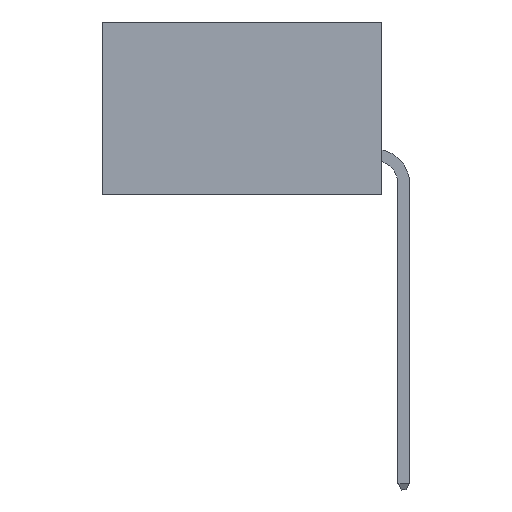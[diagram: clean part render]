
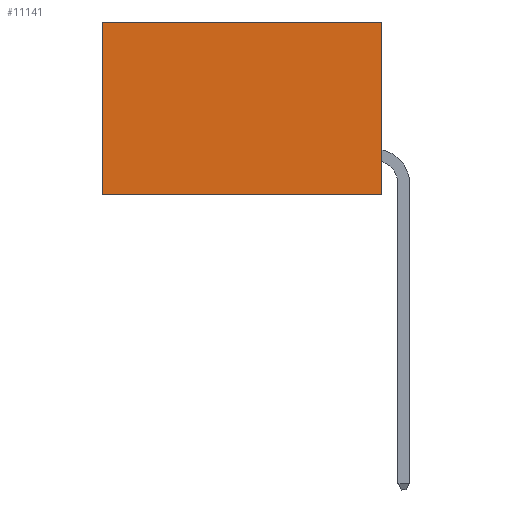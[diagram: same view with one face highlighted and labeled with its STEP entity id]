
A CAD part, left-side view. The second image highlights one B-rep face of the part: STEP entity #11141.
In plain terms, the highlighted planar face has unit normal (-1, 0, 0).
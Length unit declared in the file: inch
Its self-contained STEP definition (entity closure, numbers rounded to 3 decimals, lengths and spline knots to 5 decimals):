
#65 = ORIENTED_EDGE ( 'NONE', *, *, #1052, .F. ) ;
#114 = ORIENTED_EDGE ( 'NONE', *, *, #5266, .T. ) ;
#427 = VECTOR ( 'NONE', #7980, 39.37008 ) ;
#720 = PLANE ( 'NONE',  #4641 ) ;
#847 = CARTESIAN_POINT ( 'NONE',  ( 0.2875, 0., 0. ) ) ;
#1052 = EDGE_CURVE ( 'NONE', #8684, #6564, #4533, .T. ) ;
#1539 = EDGE_LOOP ( 'NONE', ( #114, #65, #4474, #9335 ) ) ;
#1731 = LINE ( 'NONE', #8685, #4034 ) ;
#1774 = DIRECTION ( 'NONE',  ( 1., 0., 0. ) ) ;
#2099 = FACE_OUTER_BOUND ( 'NONE', #1539, .T. ) ;
#2285 = LINE ( 'NONE', #4019, #7857 ) ;
#2439 = DIRECTION ( 'NONE',  ( 0., 0., -1. ) ) ;
#3542 = CARTESIAN_POINT ( 'NONE',  ( 0.2875, 0.6, 0. ) ) ;
#3952 = CARTESIAN_POINT ( 'NONE',  ( 0.2875, 0., -0.37 ) ) ;
#4019 = CARTESIAN_POINT ( 'NONE',  ( 0.2875, 0., 0. ) ) ;
#4034 = VECTOR ( 'NONE', #2439, 39.37008 ) ;
#4317 = CARTESIAN_POINT ( 'NONE',  ( 0.2875, 0., 0. ) ) ;
#4474 = ORIENTED_EDGE ( 'NONE', *, *, #10144, .F. ) ;
#4533 = LINE ( 'NONE', #3952, #427 ) ;
#4641 = AXIS2_PLACEMENT_3D ( 'NONE', #847, #1774, #8170 ) ;
#4711 = CARTESIAN_POINT ( 'NONE',  ( 0.2875, 0., 0. ) ) ;
#4858 = LINE ( 'NONE', #4317, #7777 ) ;
#5266 = EDGE_CURVE ( 'NONE', #8770, #6564, #1731, .T. ) ;
#6564 = VERTEX_POINT ( 'NONE', #7227 ) ;
#7227 = CARTESIAN_POINT ( 'NONE',  ( 0.2875, 0.6, -0.37 ) ) ;
#7777 = VECTOR ( 'NONE', #9662, 39.37008 ) ;
#7857 = VECTOR ( 'NONE', #11287, 39.37008 ) ;
#7980 = DIRECTION ( 'NONE',  ( 0., 1., 0. ) ) ;
#8170 = DIRECTION ( 'NONE',  ( 0., 0., -1. ) ) ;
#8684 = VERTEX_POINT ( 'NONE', #9638 ) ;
#8685 = CARTESIAN_POINT ( 'NONE',  ( 0.2875, 0.6, 0. ) ) ;
#8770 = VERTEX_POINT ( 'NONE', #3542 ) ;
#9335 = ORIENTED_EDGE ( 'NONE', *, *, #12302, .T. ) ;
#9638 = CARTESIAN_POINT ( 'NONE',  ( 0.2875, 0., -0.37 ) ) ;
#9662 = DIRECTION ( 'NONE',  ( 0., 1., 0. ) ) ;
#10144 = EDGE_CURVE ( 'NONE', #12430, #8684, #2285, .T. ) ;
#11141 = ADVANCED_FACE ( 'NONE', ( #2099 ), #720, .F. ) ;
#11287 = DIRECTION ( 'NONE',  ( 0., 0., -1. ) ) ;
#12302 = EDGE_CURVE ( 'NONE', #12430, #8770, #4858, .T. ) ;
#12430 = VERTEX_POINT ( 'NONE', #4711 ) ;
